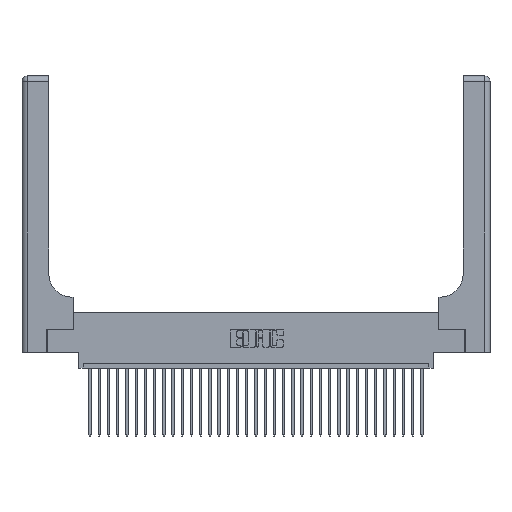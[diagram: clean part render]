
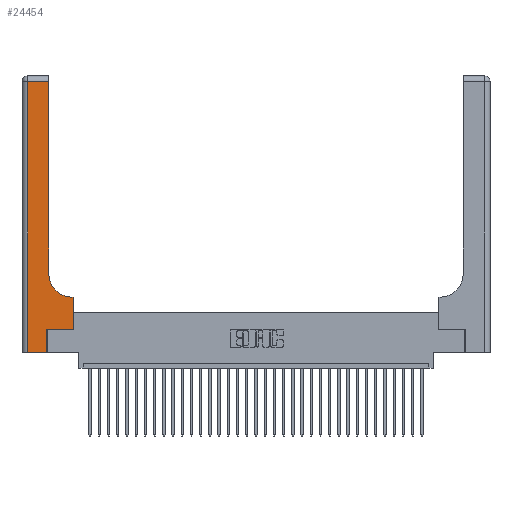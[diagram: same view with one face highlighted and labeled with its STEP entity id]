
A CAD part, top view. The second image highlights one B-rep face of the part: STEP entity #24454.
In plain terms, the highlighted planar face has unit normal (0, 0, 1).
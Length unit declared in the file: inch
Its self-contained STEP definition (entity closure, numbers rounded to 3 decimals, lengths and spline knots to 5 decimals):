
#70 = VERTEX_POINT ( 'NONE', #7999 ) ;
#890 = DIRECTION ( 'NONE',  ( -1., 0., 0. ) ) ;
#1939 = LINE ( 'NONE', #23362, #30970 ) ;
#2476 = VECTOR ( 'NONE', #3784, 39.37008 ) ;
#2651 = CARTESIAN_POINT ( 'NONE',  ( 0.06, 0., 0.37 ) ) ;
#2771 = CARTESIAN_POINT ( 'NONE',  ( 0., 2.94, 0.37 ) ) ;
#2948 = CARTESIAN_POINT ( 'NONE',  ( 0.06, 3., 0.37 ) ) ;
#3056 = DIRECTION ( 'NONE',  ( 0., 1., 0. ) ) ;
#3240 = CARTESIAN_POINT ( 'NONE',  ( 0.269, 0., 0.37 ) ) ;
#3266 = VERTEX_POINT ( 'NONE', #9547 ) ;
#3646 = ORIENTED_EDGE ( 'NONE', *, *, #13140, .T. ) ;
#3784 = DIRECTION ( 'NONE',  ( -1., 0., 0. ) ) ;
#3795 = ORIENTED_EDGE ( 'NONE', *, *, #4545, .T. ) ;
#4413 = LINE ( 'NONE', #24286, #30200 ) ;
#4545 = EDGE_CURVE ( 'NONE', #3266, #20739, #4939, .T. ) ;
#4939 = LINE ( 'NONE', #8540, #2476 ) ;
#6033 = CARTESIAN_POINT ( 'NONE',  ( 0., 3., 0.37 ) ) ;
#6598 = VERTEX_POINT ( 'NONE', #8416 ) ;
#6977 = EDGE_CURVE ( 'NONE', #70, #11554, #22724, .T. ) ;
#7167 = DIRECTION ( 'NONE',  ( 0., 0., -1. ) ) ;
#7999 = CARTESIAN_POINT ( 'NONE',  ( 0.06, 2.94, 0.37 ) ) ;
#8416 = CARTESIAN_POINT ( 'NONE',  ( 0.5585, 0.25, 0.37 ) ) ;
#8540 = CARTESIAN_POINT ( 'NONE',  ( 0.2915, 0.6, 0.37 ) ) ;
#8874 = VERTEX_POINT ( 'NONE', #17227 ) ;
#9127 = VECTOR ( 'NONE', #26596, 39.37008 ) ;
#9547 = CARTESIAN_POINT ( 'NONE',  ( 0.5585, 0.6, 0.37 ) ) ;
#9556 = VECTOR ( 'NONE', #31352, 39.37008 ) ;
#9778 = VERTEX_POINT ( 'NONE', #32929 ) ;
#9788 = LINE ( 'NONE', #10751, #14273 ) ;
#10751 = CARTESIAN_POINT ( 'NONE',  ( 0.269, 0., 0.37 ) ) ;
#11341 = DIRECTION ( 'NONE',  ( 0., 0., -1. ) ) ;
#11554 = VERTEX_POINT ( 'NONE', #2651 ) ;
#13140 = EDGE_CURVE ( 'NONE', #9778, #6598, #4413, .T. ) ;
#13653 = CARTESIAN_POINT ( 'NONE',  ( 0.5585, 0.25, 0.37 ) ) ;
#14273 = VECTOR ( 'NONE', #3056, 39.37008 ) ;
#14853 = ORIENTED_EDGE ( 'NONE', *, *, #6977, .T. ) ;
#14896 = VERTEX_POINT ( 'NONE', #3240 ) ;
#15005 = EDGE_CURVE ( 'NONE', #6598, #3266, #30471, .T. ) ;
#15347 = VECTOR ( 'NONE', #18777, 39.37008 ) ;
#15818 = FACE_OUTER_BOUND ( 'NONE', #31171, .T. ) ;
#16049 = CARTESIAN_POINT ( 'NONE',  ( 0.5415, 0.6, 0.37 ) ) ;
#17227 = CARTESIAN_POINT ( 'NONE',  ( 0.2915, 2.94, 0.37 ) ) ;
#17339 = LINE ( 'NONE', #2771, #9556 ) ;
#17441 = DIRECTION ( 'NONE',  ( 1., 0., 0. ) ) ;
#17991 = LINE ( 'NONE', #26737, #24563 ) ;
#18164 = ORIENTED_EDGE ( 'NONE', *, *, #33699, .T. ) ;
#18777 = DIRECTION ( 'NONE',  ( 0., -1., 0. ) ) ;
#19141 = CIRCLE ( 'NONE', #29826, 0.25 ) ;
#20739 = VERTEX_POINT ( 'NONE', #16049 ) ;
#20991 = CARTESIAN_POINT ( 'NONE',  ( 0.2915, 0.85, 0.37 ) ) ;
#21388 = ORIENTED_EDGE ( 'NONE', *, *, #22622, .T. ) ;
#22158 = AXIS2_PLACEMENT_3D ( 'NONE', #6033, #11341, #890 ) ;
#22622 = EDGE_CURVE ( 'NONE', #33278, #8874, #1939, .T. ) ;
#22724 = LINE ( 'NONE', #2948, #15347 ) ;
#23362 = CARTESIAN_POINT ( 'NONE',  ( 0.2915, 3., 0.37 ) ) ;
#23604 = EDGE_CURVE ( 'NONE', #14896, #9778, #9788, .T. ) ;
#24062 = ORIENTED_EDGE ( 'NONE', *, *, #15005, .T. ) ;
#24286 = CARTESIAN_POINT ( 'NONE',  ( 0.269, 0.25, 0.37 ) ) ;
#24454 = ADVANCED_FACE ( 'NONE', ( #15818 ), #26808, .F. ) ;
#24563 = VECTOR ( 'NONE', #26623, 39.37008 ) ;
#25675 = ORIENTED_EDGE ( 'NONE', *, *, #27586, .T. ) ;
#26374 = ORIENTED_EDGE ( 'NONE', *, *, #23604, .T. ) ;
#26596 = DIRECTION ( 'NONE',  ( 0., 1., 0. ) ) ;
#26623 = DIRECTION ( 'NONE',  ( 1., 0., 0. ) ) ;
#26737 = CARTESIAN_POINT ( 'NONE',  ( 0., 0., 0.37 ) ) ;
#26808 = PLANE ( 'NONE',  #22158 ) ;
#27586 = EDGE_CURVE ( 'NONE', #8874, #70, #17339, .T. ) ;
#28474 = ORIENTED_EDGE ( 'NONE', *, *, #31914, .T. ) ;
#29826 = AXIS2_PLACEMENT_3D ( 'NONE', #33123, #7167, #17441 ) ;
#30200 = VECTOR ( 'NONE', #31972, 39.37008 ) ;
#30471 = LINE ( 'NONE', #13653, #9127 ) ;
#30970 = VECTOR ( 'NONE', #31493, 39.37008 ) ;
#31171 = EDGE_LOOP ( 'NONE', ( #21388, #25675, #14853, #28474, #26374, #3646, #24062, #3795, #18164 ) ) ;
#31352 = DIRECTION ( 'NONE',  ( -1., 0., 0. ) ) ;
#31493 = DIRECTION ( 'NONE',  ( 0., 1., 0. ) ) ;
#31914 = EDGE_CURVE ( 'NONE', #11554, #14896, #17991, .T. ) ;
#31972 = DIRECTION ( 'NONE',  ( 1., 0., 0. ) ) ;
#32929 = CARTESIAN_POINT ( 'NONE',  ( 0.269, 0.25, 0.37 ) ) ;
#33123 = CARTESIAN_POINT ( 'NONE',  ( 0.5415, 0.85, 0.37 ) ) ;
#33278 = VERTEX_POINT ( 'NONE', #20991 ) ;
#33699 = EDGE_CURVE ( 'NONE', #20739, #33278, #19141, .T. ) ;
